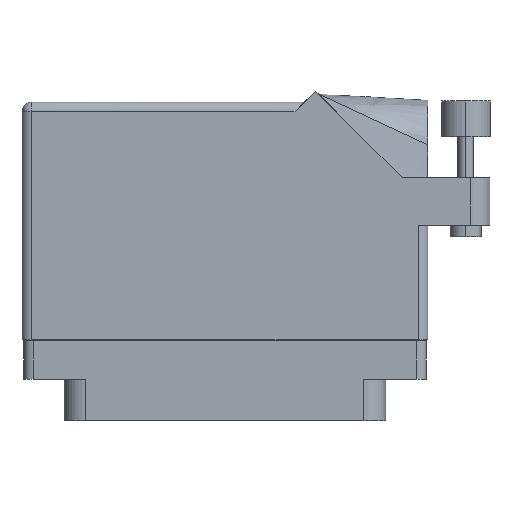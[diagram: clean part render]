
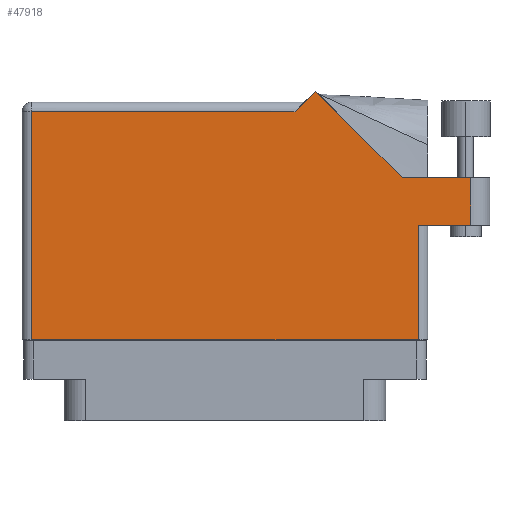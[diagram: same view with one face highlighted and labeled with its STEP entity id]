
A CAD part, front view. The second image highlights one B-rep face of the part: STEP entity #47918.
In plain terms, the highlighted face is planar.
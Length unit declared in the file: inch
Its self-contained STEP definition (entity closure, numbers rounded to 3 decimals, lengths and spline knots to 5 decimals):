
#698 = VECTOR ( 'NONE', #45580, 39.37008 ) ;
#741 = VECTOR ( 'NONE', #43679, 39.37008 ) ;
#812 = CARTESIAN_POINT ( 'NONE',  ( 1.581, 0.944, 0.455 ) ) ;
#1008 = CARTESIAN_POINT ( 'NONE',  ( 1.306, 0.637, 0.455 ) ) ;
#1599 = CARTESIAN_POINT ( 'NONE',  ( 1.14042, 0.944, 0.455 ) ) ;
#1732 = CARTESIAN_POINT ( 'NONE',  ( -1.306, 1.368, 0.455 ) ) ;
#2849 = CARTESIAN_POINT ( 'NONE',  ( -1.244, -0.1, 0.455 ) ) ;
#4407 = ORIENTED_EDGE ( 'NONE', *, *, #18295, .T. ) ;
#6021 = LINE ( 'NONE', #45086, #36903 ) ;
#6338 = LINE ( 'NONE', #37909, #698 ) ;
#12328 = CARTESIAN_POINT ( 'NONE',  ( 1.581, 0.944, 0.455 ) ) ;
#12883 = VERTEX_POINT ( 'NONE', #41714 ) ;
#13575 = VECTOR ( 'NONE', #17281, 39.37008 ) ;
#14399 = DIRECTION ( 'NONE',  ( -1., 0., 0. ) ) ;
#16313 = CARTESIAN_POINT ( 'NONE',  ( 1.14042, 0.944, 0.455 ) ) ;
#16474 = ORIENTED_EDGE ( 'NONE', *, *, #39361, .T. ) ;
#16495 = VERTEX_POINT ( 'NONE', #46872 ) ;
#17281 = DIRECTION ( 'NONE',  ( -0.707, 0.707, 0. ) ) ;
#18295 = EDGE_CURVE ( 'NONE', #33306, #29310, #46074, .T. ) ;
#18869 = CARTESIAN_POINT ( 'NONE',  ( 1.244, -0.1, 0.455 ) ) ;
#19494 = VERTEX_POINT ( 'NONE', #18869 ) ;
#20897 = LINE ( 'NONE', #51360, #48538 ) ;
#21404 = DIRECTION ( 'NONE',  ( 0., 1., 0. ) ) ;
#22242 = ORIENTED_EDGE ( 'NONE', *, *, #51204, .T. ) ;
#22635 = ORIENTED_EDGE ( 'NONE', *, *, #27833, .T. ) ;
#22925 = DIRECTION ( 'NONE',  ( 1., 0., 0. ) ) ;
#23097 = EDGE_CURVE ( 'NONE', #29706, #51554, #24291, .T. ) ;
#23498 = LINE ( 'NONE', #1008, #41081 ) ;
#23654 = DIRECTION ( 'NONE',  ( -0.707, -0.707, 0. ) ) ;
#24291 = LINE ( 'NONE', #1599, #13575 ) ;
#25045 = FACE_OUTER_BOUND ( 'NONE', #35680, .T. ) ;
#26167 = LINE ( 'NONE', #812, #33118 ) ;
#27090 = CARTESIAN_POINT ( 'NONE',  ( -1.306, -0.1, 0.455 ) ) ;
#27833 = EDGE_CURVE ( 'NONE', #19494, #12883, #6021, .T. ) ;
#27838 = EDGE_CURVE ( 'NONE', #16495, #48876, #26167, .T. ) ;
#28075 = CARTESIAN_POINT ( 'NONE',  ( 0.451, 1.368, 0.455 ) ) ;
#29310 = VERTEX_POINT ( 'NONE', #31476 ) ;
#29706 = VERTEX_POINT ( 'NONE', #16313 ) ;
#30332 = LINE ( 'NONE', #31729, #741 ) ;
#31083 = ORIENTED_EDGE ( 'NONE', *, *, #23097, .T. ) ;
#31314 = CARTESIAN_POINT ( 'NONE',  ( -1.306, 1.43, 0.455 ) ) ;
#31476 = CARTESIAN_POINT ( 'NONE',  ( -1.244, 1.368, 0.455 ) ) ;
#31529 = ORIENTED_EDGE ( 'NONE', *, *, #27838, .T. ) ;
#31602 = ORIENTED_EDGE ( 'NONE', *, *, #40645, .T. ) ;
#31729 = CARTESIAN_POINT ( 'NONE',  ( -1.244, -0.1, 0.455 ) ) ;
#33118 = VECTOR ( 'NONE', #33371, 39.37008 ) ;
#33306 = VERTEX_POINT ( 'NONE', #28075 ) ;
#33371 = DIRECTION ( 'NONE',  ( 0., 1., 0. ) ) ;
#33888 = ORIENTED_EDGE ( 'NONE', *, *, #46011, .T. ) ;
#34188 = VECTOR ( 'NONE', #14399, 39.37008 ) ;
#34648 = VECTOR ( 'NONE', #22925, 39.37008 ) ;
#35194 = DIRECTION ( 'NONE',  ( -1., 0., 0. ) ) ;
#35314 = AXIS2_PLACEMENT_3D ( 'NONE', #31314, #47589, #35194 ) ;
#35680 = EDGE_LOOP ( 'NONE', ( #16474, #31529, #33888, #31083, #36532, #4407, #22242, #31602, #22635 ) ) ;
#36532 = ORIENTED_EDGE ( 'NONE', *, *, #51220, .T. ) ;
#36903 = VECTOR ( 'NONE', #21404, 39.37008 ) ;
#37909 = CARTESIAN_POINT ( 'NONE',  ( 1.706, 0.944, 0.455 ) ) ;
#39361 = EDGE_CURVE ( 'NONE', #12883, #16495, #23498, .T. ) ;
#39579 = PLANE ( 'NONE',  #35314 ) ;
#40645 = EDGE_CURVE ( 'NONE', #44609, #19494, #45272, .T. ) ;
#41081 = VECTOR ( 'NONE', #44625, 39.37008 ) ;
#41714 = CARTESIAN_POINT ( 'NONE',  ( 1.244, 0.637, 0.455 ) ) ;
#43679 = DIRECTION ( 'NONE',  ( 0., -1., 0. ) ) ;
#44609 = VERTEX_POINT ( 'NONE', #2849 ) ;
#44625 = DIRECTION ( 'NONE',  ( 1., 0., 0. ) ) ;
#45086 = CARTESIAN_POINT ( 'NONE',  ( 1.244, 0.637, 0.455 ) ) ;
#45272 = LINE ( 'NONE', #27090, #34648 ) ;
#45580 = DIRECTION ( 'NONE',  ( -1., 0., 0. ) ) ;
#46011 = EDGE_CURVE ( 'NONE', #48876, #29706, #6338, .T. ) ;
#46074 = LINE ( 'NONE', #1732, #34188 ) ;
#46209 = CARTESIAN_POINT ( 'NONE',  ( 0.58371, 1.50071, 0.455 ) ) ;
#46872 = CARTESIAN_POINT ( 'NONE',  ( 1.581, 0.637, 0.455 ) ) ;
#47589 = DIRECTION ( 'NONE',  ( 0., 0., -1. ) ) ;
#47918 = ADVANCED_FACE ( 'NONE', ( #25045 ), #39579, .F. ) ;
#48538 = VECTOR ( 'NONE', #23654, 39.37008 ) ;
#48876 = VERTEX_POINT ( 'NONE', #12328 ) ;
#51204 = EDGE_CURVE ( 'NONE', #29310, #44609, #30332, .T. ) ;
#51220 = EDGE_CURVE ( 'NONE', #51554, #33306, #20897, .T. ) ;
#51360 = CARTESIAN_POINT ( 'NONE',  ( 0.513, 1.43, 0.455 ) ) ;
#51554 = VERTEX_POINT ( 'NONE', #46209 ) ;
